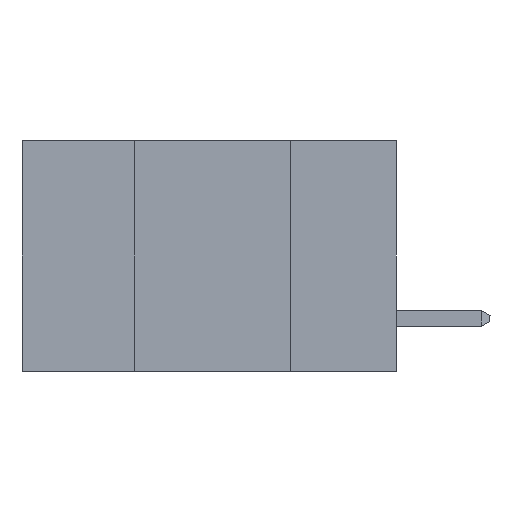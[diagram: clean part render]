
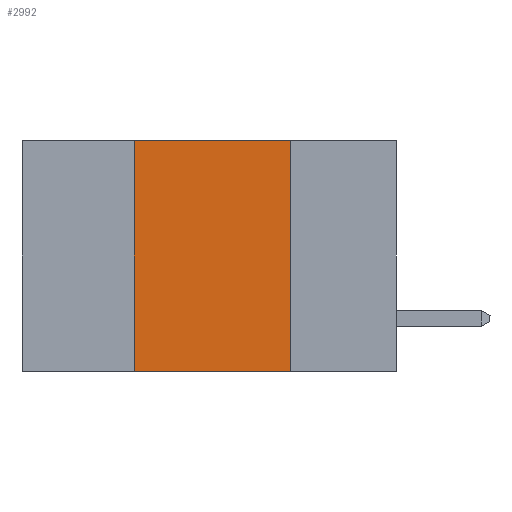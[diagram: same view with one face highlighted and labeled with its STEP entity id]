
A CAD part, left-side view. The second image highlights one B-rep face of the part: STEP entity #2992.
In plain terms, the highlighted planar face has unit normal (-1, 0, 0).
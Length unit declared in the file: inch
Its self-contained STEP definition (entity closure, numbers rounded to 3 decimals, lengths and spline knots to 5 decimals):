
#77 = LINE ( 'NONE', #3101, #1324 ) ;
#95 = AXIS2_PLACEMENT_3D ( 'NONE', #112, #11945, #10672 ) ;
#112 = CARTESIAN_POINT ( 'NONE',  ( 0., 0.6, 0. ) ) ;
#736 = DIRECTION ( 'NONE',  ( 0., -1., 0. ) ) ;
#1014 = DIRECTION ( 'NONE',  ( 0., -1., 0. ) ) ;
#1295 = VECTOR ( 'NONE', #736, 39.37008 ) ;
#1324 = VECTOR ( 'NONE', #12918, 39.37008 ) ;
#1576 = CARTESIAN_POINT ( 'NONE',  ( 0., 0.17, -0.37 ) ) ;
#2865 = CARTESIAN_POINT ( 'NONE',  ( 0., 0.17, 0. ) ) ;
#2992 = ADVANCED_FACE ( 'NONE', ( #14000 ), #13088, .F. ) ;
#3055 = ORIENTED_EDGE ( 'NONE', *, *, #10866, .T. ) ;
#3101 = CARTESIAN_POINT ( 'NONE',  ( 0., 0.42, -0.37 ) ) ;
#3947 = EDGE_LOOP ( 'NONE', ( #12021, #7904, #7408, #3055 ) ) ;
#4819 = EDGE_CURVE ( 'NONE', #10285, #5848, #9385, .T. ) ;
#5134 = CARTESIAN_POINT ( 'NONE',  ( 0., 0.6, 0. ) ) ;
#5848 = VERTEX_POINT ( 'NONE', #11150 ) ;
#7073 = LINE ( 'NONE', #5134, #1295 ) ;
#7408 = ORIENTED_EDGE ( 'NONE', *, *, #13138, .F. ) ;
#7750 = VERTEX_POINT ( 'NONE', #8893 ) ;
#7904 = ORIENTED_EDGE ( 'NONE', *, *, #9427, .F. ) ;
#8893 = CARTESIAN_POINT ( 'NONE',  ( 0., 0.42, 0. ) ) ;
#9114 = VECTOR ( 'NONE', #10240, 39.37008 ) ;
#9385 = LINE ( 'NONE', #1576, #9114 ) ;
#9427 = EDGE_CURVE ( 'NONE', #7750, #10285, #7073, .T. ) ;
#9553 = CARTESIAN_POINT ( 'NONE',  ( 0., 0.42, -0.37 ) ) ;
#9745 = CARTESIAN_POINT ( 'NONE',  ( 0., 0.6, -0.37 ) ) ;
#10240 = DIRECTION ( 'NONE',  ( 0., 0., -1. ) ) ;
#10285 = VERTEX_POINT ( 'NONE', #2865 ) ;
#10287 = VERTEX_POINT ( 'NONE', #9553 ) ;
#10667 = LINE ( 'NONE', #9745, #11288 ) ;
#10672 = DIRECTION ( 'NONE',  ( 0., 0., -1. ) ) ;
#10866 = EDGE_CURVE ( 'NONE', #10287, #5848, #10667, .T. ) ;
#11150 = CARTESIAN_POINT ( 'NONE',  ( 0., 0.17, -0.37 ) ) ;
#11288 = VECTOR ( 'NONE', #1014, 39.37008 ) ;
#11945 = DIRECTION ( 'NONE',  ( 1., 0., 0. ) ) ;
#12021 = ORIENTED_EDGE ( 'NONE', *, *, #4819, .F. ) ;
#12918 = DIRECTION ( 'NONE',  ( 0., 0., 1. ) ) ;
#13088 = PLANE ( 'NONE',  #95 ) ;
#13138 = EDGE_CURVE ( 'NONE', #10287, #7750, #77, .T. ) ;
#14000 = FACE_OUTER_BOUND ( 'NONE', #3947, .T. ) ;
